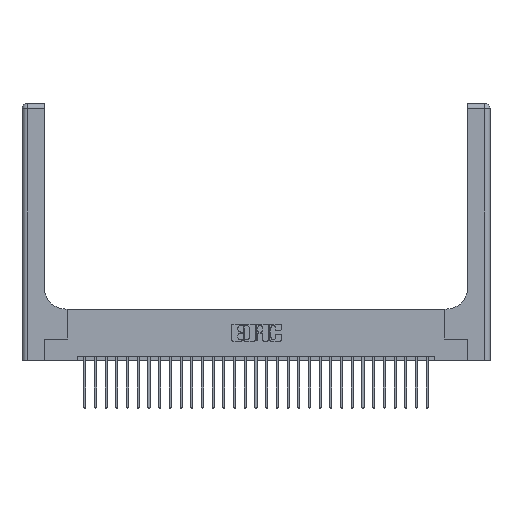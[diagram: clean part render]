
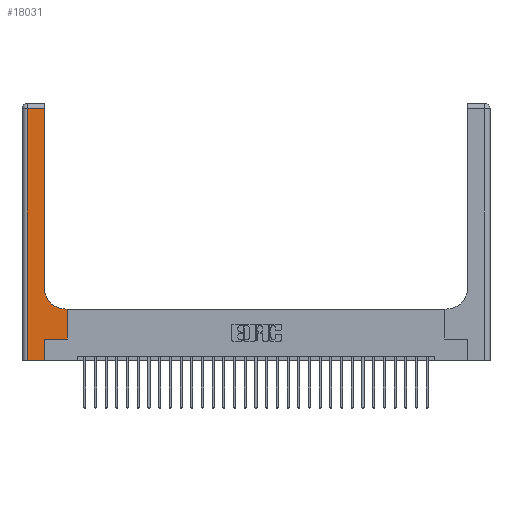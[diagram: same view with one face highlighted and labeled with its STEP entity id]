
A CAD part, top view. The second image highlights one B-rep face of the part: STEP entity #18031.
In plain terms, the highlighted planar face has unit normal (0, 0, 1).
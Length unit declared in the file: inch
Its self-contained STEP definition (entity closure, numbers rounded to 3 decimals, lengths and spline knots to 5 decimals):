
#182 = VERTEX_POINT ( 'NONE', #19466 ) ;
#783 = LINE ( 'NONE', #12193, #4534 ) ;
#853 = LINE ( 'NONE', #17476, #22403 ) ;
#947 = DIRECTION ( 'NONE',  ( 1., 0., 0. ) ) ;
#1983 = CARTESIAN_POINT ( 'NONE',  ( 0., 2.94, 0.37 ) ) ;
#2296 = ORIENTED_EDGE ( 'NONE', *, *, #25065, .T. ) ;
#2988 = LINE ( 'NONE', #4147, #3994 ) ;
#3095 = EDGE_CURVE ( 'NONE', #5922, #27083, #27607, .T. ) ;
#3994 = VECTOR ( 'NONE', #24110, 39.37008 ) ;
#4147 = CARTESIAN_POINT ( 'NONE',  ( 0.528, 0.25, 0.37 ) ) ;
#4246 = DIRECTION ( 'NONE',  ( -1., 0., 0. ) ) ;
#4534 = VECTOR ( 'NONE', #5666, 39.37008 ) ;
#4663 = EDGE_CURVE ( 'NONE', #7304, #182, #8533, .T. ) ;
#5132 = DIRECTION ( 'NONE',  ( 0., -1., 0. ) ) ;
#5666 = DIRECTION ( 'NONE',  ( 0., 1., 0. ) ) ;
#5683 = CARTESIAN_POINT ( 'NONE',  ( 0.265, 0., 0.37 ) ) ;
#5922 = VERTEX_POINT ( 'NONE', #14760 ) ;
#5996 = AXIS2_PLACEMENT_3D ( 'NONE', #13342, #15556, #11861 ) ;
#6553 = EDGE_CURVE ( 'NONE', #13574, #10584, #2988, .T. ) ;
#6571 = CARTESIAN_POINT ( 'NONE',  ( 0., 3., 0.37 ) ) ;
#7258 = FACE_OUTER_BOUND ( 'NONE', #22490, .T. ) ;
#7304 = VERTEX_POINT ( 'NONE', #12350 ) ;
#8481 = DIRECTION ( 'NONE',  ( -1., 0., 0. ) ) ;
#8533 = CIRCLE ( 'NONE', #5996, 0.25 ) ;
#8871 = LINE ( 'NONE', #25161, #22585 ) ;
#9792 = ORIENTED_EDGE ( 'NONE', *, *, #14818, .T. ) ;
#10213 = AXIS2_PLACEMENT_3D ( 'NONE', #6571, #24033, #4246 ) ;
#10584 = VERTEX_POINT ( 'NONE', #15421 ) ;
#10821 = CARTESIAN_POINT ( 'NONE',  ( 0.528, 0.25, 0.37 ) ) ;
#11635 = CARTESIAN_POINT ( 'NONE',  ( 0.06, 2.94, 0.37 ) ) ;
#11861 = DIRECTION ( 'NONE',  ( 1., 0., 0. ) ) ;
#12193 = CARTESIAN_POINT ( 'NONE',  ( 0.26, 3., 0.37 ) ) ;
#12350 = CARTESIAN_POINT ( 'NONE',  ( 0.51, 0.6, 0.37 ) ) ;
#12810 = VECTOR ( 'NONE', #24888, 39.37008 ) ;
#13342 = CARTESIAN_POINT ( 'NONE',  ( 0.51, 0.85, 0.37 ) ) ;
#13574 = VERTEX_POINT ( 'NONE', #10821 ) ;
#13630 = DIRECTION ( 'NONE',  ( 1., 0., 0. ) ) ;
#13984 = EDGE_CURVE ( 'NONE', #10584, #7304, #8871, .T. ) ;
#14074 = VERTEX_POINT ( 'NONE', #15210 ) ;
#14447 = CARTESIAN_POINT ( 'NONE',  ( 0.265, 0.25, 0.37 ) ) ;
#14760 = CARTESIAN_POINT ( 'NONE',  ( 0.26, 2.94, 0.37 ) ) ;
#14818 = EDGE_CURVE ( 'NONE', #27083, #15011, #18147, .T. ) ;
#15011 = VERTEX_POINT ( 'NONE', #25259 ) ;
#15210 = CARTESIAN_POINT ( 'NONE',  ( 0.265, 0., 0.37 ) ) ;
#15421 = CARTESIAN_POINT ( 'NONE',  ( 0.528, 0.6, 0.37 ) ) ;
#15556 = DIRECTION ( 'NONE',  ( 0., 0., -1. ) ) ;
#15867 = CARTESIAN_POINT ( 'NONE',  ( 0.06, 3., 0.37 ) ) ;
#15943 = ORIENTED_EDGE ( 'NONE', *, *, #13984, .T. ) ;
#16494 = ORIENTED_EDGE ( 'NONE', *, *, #22908, .T. ) ;
#17476 = CARTESIAN_POINT ( 'NONE',  ( 0.265, 0.25, 0.37 ) ) ;
#18031 = ADVANCED_FACE ( 'NONE', ( #7258 ), #21757, .F. ) ;
#18147 = LINE ( 'NONE', #15867, #19156 ) ;
#19156 = VECTOR ( 'NONE', #5132, 39.37008 ) ;
#19466 = CARTESIAN_POINT ( 'NONE',  ( 0.26, 0.85, 0.37 ) ) ;
#20518 = ORIENTED_EDGE ( 'NONE', *, *, #20875, .T. ) ;
#20875 = EDGE_CURVE ( 'NONE', #14074, #22648, #26919, .T. ) ;
#20954 = ORIENTED_EDGE ( 'NONE', *, *, #25004, .T. ) ;
#21060 = ORIENTED_EDGE ( 'NONE', *, *, #6553, .T. ) ;
#21131 = ORIENTED_EDGE ( 'NONE', *, *, #4663, .T. ) ;
#21345 = ORIENTED_EDGE ( 'NONE', *, *, #3095, .T. ) ;
#21757 = PLANE ( 'NONE',  #10213 ) ;
#22403 = VECTOR ( 'NONE', #13630, 39.37008 ) ;
#22490 = EDGE_LOOP ( 'NONE', ( #2296, #21345, #9792, #20954, #20518, #16494, #21060, #15943, #21131 ) ) ;
#22585 = VECTOR ( 'NONE', #27335, 39.37008 ) ;
#22648 = VERTEX_POINT ( 'NONE', #14447 ) ;
#22908 = EDGE_CURVE ( 'NONE', #22648, #13574, #853, .T. ) ;
#23187 = VECTOR ( 'NONE', #8481, 39.37008 ) ;
#24033 = DIRECTION ( 'NONE',  ( 0., 0., -1. ) ) ;
#24110 = DIRECTION ( 'NONE',  ( 0., 1., 0. ) ) ;
#24888 = DIRECTION ( 'NONE',  ( 0., 1., 0. ) ) ;
#25004 = EDGE_CURVE ( 'NONE', #15011, #14074, #27822, .T. ) ;
#25065 = EDGE_CURVE ( 'NONE', #182, #5922, #783, .T. ) ;
#25161 = CARTESIAN_POINT ( 'NONE',  ( 0.26, 0.6, 0.37 ) ) ;
#25259 = CARTESIAN_POINT ( 'NONE',  ( 0.06, 0., 0.37 ) ) ;
#25773 = VECTOR ( 'NONE', #947, 39.37008 ) ;
#26787 = CARTESIAN_POINT ( 'NONE',  ( 0., 0., 0.37 ) ) ;
#26919 = LINE ( 'NONE', #5683, #12810 ) ;
#27083 = VERTEX_POINT ( 'NONE', #11635 ) ;
#27335 = DIRECTION ( 'NONE',  ( -1., 0., 0. ) ) ;
#27607 = LINE ( 'NONE', #1983, #23187 ) ;
#27822 = LINE ( 'NONE', #26787, #25773 ) ;
